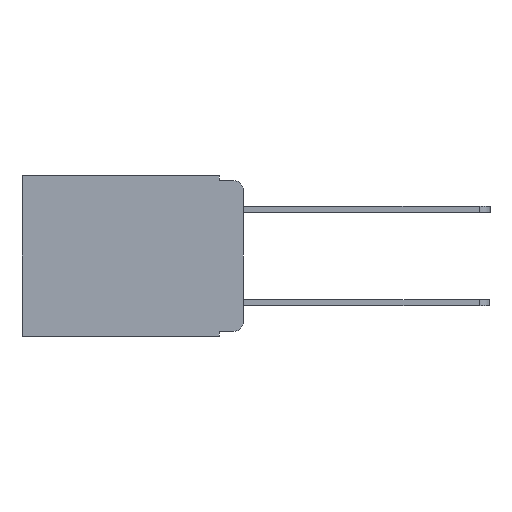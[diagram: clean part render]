
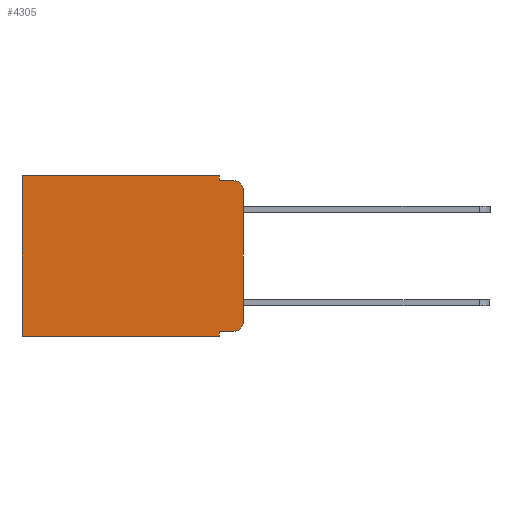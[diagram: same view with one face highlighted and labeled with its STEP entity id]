
A CAD part, left-side view. The second image highlights one B-rep face of the part: STEP entity #4305.
In plain terms, the highlighted planar face has unit normal (-1, 0, 0).
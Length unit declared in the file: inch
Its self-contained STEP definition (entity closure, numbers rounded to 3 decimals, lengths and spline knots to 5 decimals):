
#171 = CARTESIAN_POINT ( 'NONE',  ( 0.298, 0.02, -0.03 ) ) ;
#221 = LINE ( 'NONE', #3678, #5860 ) ;
#1134 = VECTOR ( 'NONE', #12548, 39.37008 ) ;
#1314 = DIRECTION ( 'NONE',  ( 0., 0., -1. ) ) ;
#1317 = CARTESIAN_POINT ( 'NONE',  ( 0.298, 0.02, -0.333 ) ) ;
#1703 = EDGE_CURVE ( 'NONE', #2228, #10338, #9235, .T. ) ;
#1768 = CARTESIAN_POINT ( 'NONE',  ( 0.298, 0.051, 0. ) ) ;
#1800 = EDGE_CURVE ( 'NONE', #4524, #10338, #221, .T. ) ;
#1912 = PLANE ( 'NONE',  #7673 ) ;
#2228 = VERTEX_POINT ( 'NONE', #8414 ) ;
#2458 = CARTESIAN_POINT ( 'NONE',  ( 0.298, 0.051, -0.01 ) ) ;
#2533 = EDGE_CURVE ( 'NONE', #6199, #8176, #8421, .T. ) ;
#3014 = DIRECTION ( 'NONE',  ( 1., 0., 0. ) ) ;
#3247 = VERTEX_POINT ( 'NONE', #7230 ) ;
#3277 = EDGE_CURVE ( 'NONE', #8176, #4095, #10809, .T. ) ;
#3313 = CIRCLE ( 'NONE', #8121, 0.02 ) ;
#3324 = VERTEX_POINT ( 'NONE', #1317 ) ;
#3507 = VECTOR ( 'NONE', #11409, 39.37008 ) ;
#3643 = EDGE_LOOP ( 'NONE', ( #3879, #5656, #6452, #7014, #6462, #6302, #12847, #12745, #12837, #7479 ) ) ;
#3660 = VECTOR ( 'NONE', #6670, 39.37008 ) ;
#3678 = CARTESIAN_POINT ( 'NONE',  ( 0.298, 0.473, 0. ) ) ;
#3879 = ORIENTED_EDGE ( 'NONE', *, *, #6329, .F. ) ;
#4056 = LINE ( 'NONE', #1768, #1134 ) ;
#4095 = VERTEX_POINT ( 'NONE', #10429 ) ;
#4305 = ADVANCED_FACE ( 'NONE', ( #9045 ), #1912, .F. ) ;
#4327 = VECTOR ( 'NONE', #7662, 39.37008 ) ;
#4524 = VERTEX_POINT ( 'NONE', #4762 ) ;
#4762 = CARTESIAN_POINT ( 'NONE',  ( 0.298, 0.473, 0. ) ) ;
#4831 = EDGE_CURVE ( 'NONE', #3247, #4095, #8524, .T. ) ;
#5064 = LINE ( 'NONE', #11185, #12715 ) ;
#5065 = DIRECTION ( 'NONE',  ( -1., 0., 0. ) ) ;
#5157 = CARTESIAN_POINT ( 'NONE',  ( 0.298, 0.051, -0.333 ) ) ;
#5162 = CARTESIAN_POINT ( 'NONE',  ( 0.298, 0., -0.313 ) ) ;
#5656 = ORIENTED_EDGE ( 'NONE', *, *, #4831, .T. ) ;
#5762 = DIRECTION ( 'NONE',  ( 0., 1., 0. ) ) ;
#5860 = VECTOR ( 'NONE', #6886, 39.37008 ) ;
#6199 = VERTEX_POINT ( 'NONE', #9311 ) ;
#6272 = DIRECTION ( 'NONE',  ( 0., 0., -1. ) ) ;
#6277 = CARTESIAN_POINT ( 'NONE',  ( 0.298, 0.051, 0. ) ) ;
#6302 = ORIENTED_EDGE ( 'NONE', *, *, #1800, .T. ) ;
#6329 = EDGE_CURVE ( 'NONE', #3247, #8286, #7214, .T. ) ;
#6383 = CARTESIAN_POINT ( 'NONE',  ( 0.298, 0., 0. ) ) ;
#6452 = ORIENTED_EDGE ( 'NONE', *, *, #3277, .F. ) ;
#6462 = ORIENTED_EDGE ( 'NONE', *, *, #7018, .T. ) ;
#6483 = CARTESIAN_POINT ( 'NONE',  ( 0.298, 0.473, -0.343 ) ) ;
#6565 = VECTOR ( 'NONE', #8139, 39.37008 ) ;
#6670 = DIRECTION ( 'NONE',  ( 0., -1., 0. ) ) ;
#6886 = DIRECTION ( 'NONE',  ( 0., 0., -1. ) ) ;
#7014 = ORIENTED_EDGE ( 'NONE', *, *, #2533, .F. ) ;
#7018 = EDGE_CURVE ( 'NONE', #6199, #4524, #5064, .T. ) ;
#7214 = LINE ( 'NONE', #10285, #4327 ) ;
#7230 = CARTESIAN_POINT ( 'NONE',  ( 0.298, 0., -0.03 ) ) ;
#7479 = ORIENTED_EDGE ( 'NONE', *, *, #10742, .T. ) ;
#7642 = CARTESIAN_POINT ( 'NONE',  ( 0.298, 0.051, -0.333 ) ) ;
#7662 = DIRECTION ( 'NONE',  ( 0., 0., -1. ) ) ;
#7673 = AXIS2_PLACEMENT_3D ( 'NONE', #6383, #3014, #10033 ) ;
#7801 = DIRECTION ( 'NONE',  ( -1., 0., 0. ) ) ;
#8052 = VERTEX_POINT ( 'NONE', #7642 ) ;
#8121 = AXIS2_PLACEMENT_3D ( 'NONE', #10669, #5065, #11536 ) ;
#8139 = DIRECTION ( 'NONE',  ( 0., -1., 0. ) ) ;
#8176 = VERTEX_POINT ( 'NONE', #2458 ) ;
#8286 = VERTEX_POINT ( 'NONE', #5162 ) ;
#8414 = CARTESIAN_POINT ( 'NONE',  ( 0.298, 0.051, -0.343 ) ) ;
#8421 = LINE ( 'NONE', #6277, #12779 ) ;
#8524 = CIRCLE ( 'NONE', #11423, 0.02 ) ;
#8983 = LINE ( 'NONE', #5157, #6565 ) ;
#9045 = FACE_OUTER_BOUND ( 'NONE', #3643, .T. ) ;
#9235 = LINE ( 'NONE', #12069, #3507 ) ;
#9311 = CARTESIAN_POINT ( 'NONE',  ( 0.298, 0.051, 0. ) ) ;
#10033 = DIRECTION ( 'NONE',  ( 0., 0., -1. ) ) ;
#10285 = CARTESIAN_POINT ( 'NONE',  ( 0.298, 0., 0. ) ) ;
#10338 = VERTEX_POINT ( 'NONE', #6483 ) ;
#10429 = CARTESIAN_POINT ( 'NONE',  ( 0.298, 0.02, -0.01 ) ) ;
#10669 = CARTESIAN_POINT ( 'NONE',  ( 0.298, 0.02, -0.313 ) ) ;
#10742 = EDGE_CURVE ( 'NONE', #3324, #8286, #3313, .T. ) ;
#10809 = LINE ( 'NONE', #11178, #3660 ) ;
#11178 = CARTESIAN_POINT ( 'NONE',  ( 0.298, 0.051, -0.01 ) ) ;
#11185 = CARTESIAN_POINT ( 'NONE',  ( 0.298, 0., 0. ) ) ;
#11409 = DIRECTION ( 'NONE',  ( 0., 1., 0. ) ) ;
#11423 = AXIS2_PLACEMENT_3D ( 'NONE', #171, #7801, #1314 ) ;
#11536 = DIRECTION ( 'NONE',  ( 0., 0., -1. ) ) ;
#11937 = EDGE_CURVE ( 'NONE', #8052, #3324, #8983, .T. ) ;
#12069 = CARTESIAN_POINT ( 'NONE',  ( 0.298, 0., -0.343 ) ) ;
#12533 = EDGE_CURVE ( 'NONE', #8052, #2228, #4056, .T. ) ;
#12548 = DIRECTION ( 'NONE',  ( 0., 0., -1. ) ) ;
#12715 = VECTOR ( 'NONE', #5762, 39.37008 ) ;
#12745 = ORIENTED_EDGE ( 'NONE', *, *, #12533, .F. ) ;
#12779 = VECTOR ( 'NONE', #6272, 39.37008 ) ;
#12837 = ORIENTED_EDGE ( 'NONE', *, *, #11937, .T. ) ;
#12847 = ORIENTED_EDGE ( 'NONE', *, *, #1703, .F. ) ;
